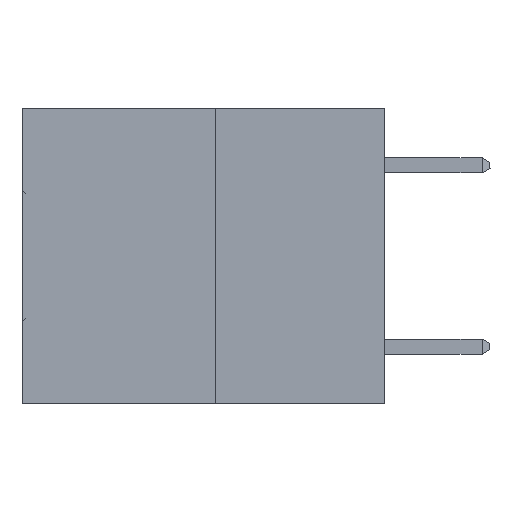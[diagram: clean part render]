
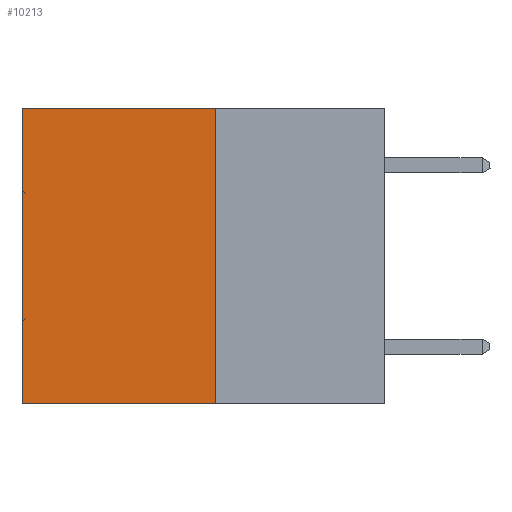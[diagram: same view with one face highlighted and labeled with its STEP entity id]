
A CAD part, left-side view. The second image highlights one B-rep face of the part: STEP entity #10213.
In plain terms, the highlighted planar face has unit normal (-1, 0, 0).
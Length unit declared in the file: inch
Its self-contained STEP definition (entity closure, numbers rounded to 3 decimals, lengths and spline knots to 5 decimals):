
#314 = VERTEX_POINT ( 'NONE', #26362 ) ;
#400 = DIRECTION ( 'NONE',  ( 0., 1., 0. ) ) ;
#2297 = ORIENTED_EDGE ( 'NONE', *, *, #24738, .T. ) ;
#2349 = VERTEX_POINT ( 'NONE', #20522 ) ;
#2947 = ORIENTED_EDGE ( 'NONE', *, *, #9944, .F. ) ;
#3112 = CARTESIAN_POINT ( 'NONE',  ( 0.3165, 0.28, -0.49 ) ) ;
#4222 = ORIENTED_EDGE ( 'NONE', *, *, #7312, .T. ) ;
#4480 = VECTOR ( 'NONE', #28195, 39.37008 ) ;
#4981 = DIRECTION ( 'NONE',  ( 1., 0., 0. ) ) ;
#7312 = EDGE_CURVE ( 'NONE', #314, #26718, #32316, .T. ) ;
#7393 = LINE ( 'NONE', #29480, #34700 ) ;
#8579 = CARTESIAN_POINT ( 'NONE',  ( 0.3165, 0.6, 0. ) ) ;
#9114 = CARTESIAN_POINT ( 'NONE',  ( 0.3165, 0.28, -0.49 ) ) ;
#9944 = EDGE_CURVE ( 'NONE', #314, #30292, #7393, .T. ) ;
#10213 = ADVANCED_FACE ( 'NONE', ( #10318 ), #21137, .F. ) ;
#10318 = FACE_OUTER_BOUND ( 'NONE', #10581, .T. ) ;
#10447 = CARTESIAN_POINT ( 'NONE',  ( 0.3165, 0.6, -0.49 ) ) ;
#10581 = EDGE_LOOP ( 'NONE', ( #2297, #30340, #2947, #4222 ) ) ;
#11109 = CARTESIAN_POINT ( 'NONE',  ( 0.3165, 0.28, 0. ) ) ;
#14544 = LINE ( 'NONE', #10447, #20487 ) ;
#20487 = VECTOR ( 'NONE', #24117, 39.37008 ) ;
#20522 = CARTESIAN_POINT ( 'NONE',  ( 0.3165, 0.6, -0.49 ) ) ;
#21015 = CARTESIAN_POINT ( 'NONE',  ( 0.3165, 0.28, -0.49 ) ) ;
#21137 = PLANE ( 'NONE',  #35220 ) ;
#24117 = DIRECTION ( 'NONE',  ( 0., 0., -1. ) ) ;
#24738 = EDGE_CURVE ( 'NONE', #26718, #2349, #14544, .T. ) ;
#25053 = VECTOR ( 'NONE', #400, 39.37008 ) ;
#26362 = CARTESIAN_POINT ( 'NONE',  ( 0.3165, 0.28, 0. ) ) ;
#26718 = VERTEX_POINT ( 'NONE', #8579 ) ;
#28195 = DIRECTION ( 'NONE',  ( 0., 1., 0. ) ) ;
#29249 = DIRECTION ( 'NONE',  ( 0., 0., -1. ) ) ;
#29480 = CARTESIAN_POINT ( 'NONE',  ( 0.3165, 0.28, -0.49 ) ) ;
#30292 = VERTEX_POINT ( 'NONE', #3112 ) ;
#30340 = ORIENTED_EDGE ( 'NONE', *, *, #34291, .F. ) ;
#31893 = DIRECTION ( 'NONE',  ( 0., 0., -1. ) ) ;
#32316 = LINE ( 'NONE', #11109, #25053 ) ;
#34291 = EDGE_CURVE ( 'NONE', #30292, #2349, #34737, .T. ) ;
#34700 = VECTOR ( 'NONE', #31893, 39.37008 ) ;
#34737 = LINE ( 'NONE', #9114, #4480 ) ;
#35220 = AXIS2_PLACEMENT_3D ( 'NONE', #21015, #4981, #29249 ) ;
